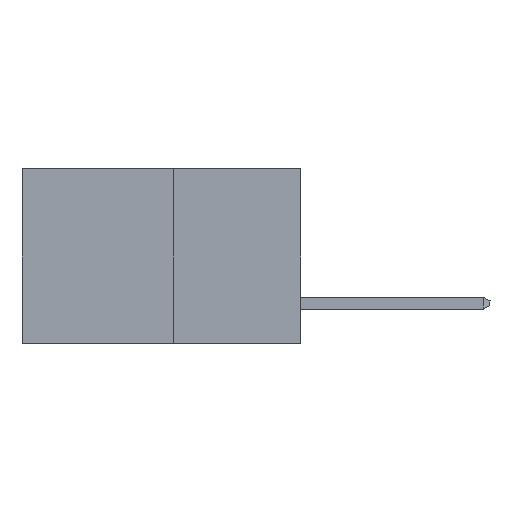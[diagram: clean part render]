
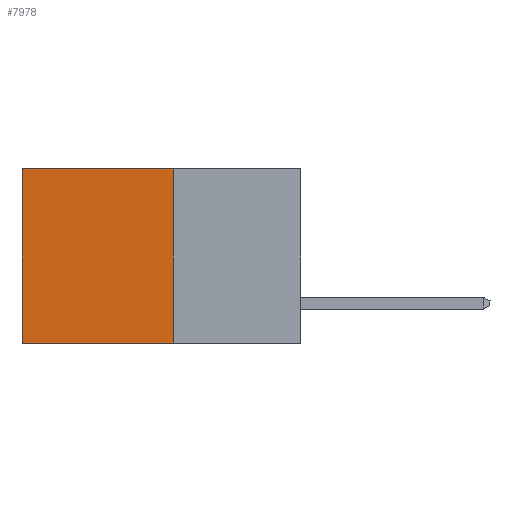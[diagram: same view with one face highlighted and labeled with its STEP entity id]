
A CAD part, left-side view. The second image highlights one B-rep face of the part: STEP entity #7978.
In plain terms, the highlighted planar face has unit normal (-1, 0, 0).
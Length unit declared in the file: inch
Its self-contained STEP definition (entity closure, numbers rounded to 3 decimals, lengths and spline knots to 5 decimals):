
#73 = DIRECTION ( 'NONE',  ( 0., 0., -1. ) ) ;
#95 = EDGE_CURVE ( 'NONE', #4328, #338, #3248, .T. ) ;
#338 = VERTEX_POINT ( 'NONE', #5758 ) ;
#767 = CARTESIAN_POINT ( 'NONE',  ( 0.277, 0.27, 0. ) ) ;
#974 = VERTEX_POINT ( 'NONE', #5939 ) ;
#1022 = LINE ( 'NONE', #767, #6260 ) ;
#1115 = LINE ( 'NONE', #7051, #4926 ) ;
#1718 = VERTEX_POINT ( 'NONE', #2496 ) ;
#2496 = CARTESIAN_POINT ( 'NONE',  ( 0.277, 0.59, 0. ) ) ;
#2800 = ORIENTED_EDGE ( 'NONE', *, *, #3115, .F. ) ;
#3115 = EDGE_CURVE ( 'NONE', #974, #4328, #1115, .T. ) ;
#3248 = LINE ( 'NONE', #6952, #6782 ) ;
#3275 = FACE_OUTER_BOUND ( 'NONE', #4754, .T. ) ;
#3795 = ORIENTED_EDGE ( 'NONE', *, *, #7130, .T. ) ;
#3857 = PLANE ( 'NONE',  #6784 ) ;
#4147 = CARTESIAN_POINT ( 'NONE',  ( 0.277, 0.59, -0.37 ) ) ;
#4328 = VERTEX_POINT ( 'NONE', #5882 ) ;
#4445 = ORIENTED_EDGE ( 'NONE', *, *, #8864, .T. ) ;
#4510 = VECTOR ( 'NONE', #6279, 39.37008 ) ;
#4560 = DIRECTION ( 'NONE',  ( 0., 0., -1. ) ) ;
#4754 = EDGE_LOOP ( 'NONE', ( #3795, #5561, #2800, #4445 ) ) ;
#4926 = VECTOR ( 'NONE', #73, 39.37008 ) ;
#5561 = ORIENTED_EDGE ( 'NONE', *, *, #95, .F. ) ;
#5758 = CARTESIAN_POINT ( 'NONE',  ( 0.277, 0.59, -0.37 ) ) ;
#5882 = CARTESIAN_POINT ( 'NONE',  ( 0.277, 0.27, -0.37 ) ) ;
#5939 = CARTESIAN_POINT ( 'NONE',  ( 0.277, 0.27, 0. ) ) ;
#5952 = CARTESIAN_POINT ( 'NONE',  ( 0.277, 0.27, -0.37 ) ) ;
#6260 = VECTOR ( 'NONE', #7828, 39.37008 ) ;
#6279 = DIRECTION ( 'NONE',  ( 0., 0., -1. ) ) ;
#6382 = LINE ( 'NONE', #4147, #4510 ) ;
#6782 = VECTOR ( 'NONE', #7094, 39.37008 ) ;
#6784 = AXIS2_PLACEMENT_3D ( 'NONE', #5952, #8725, #4560 ) ;
#6952 = CARTESIAN_POINT ( 'NONE',  ( 0.277, 0.27, -0.37 ) ) ;
#7051 = CARTESIAN_POINT ( 'NONE',  ( 0.277, 0.27, -0.37 ) ) ;
#7094 = DIRECTION ( 'NONE',  ( 0., 1., 0. ) ) ;
#7130 = EDGE_CURVE ( 'NONE', #1718, #338, #6382, .T. ) ;
#7828 = DIRECTION ( 'NONE',  ( 0., 1., 0. ) ) ;
#7978 = ADVANCED_FACE ( 'NONE', ( #3275 ), #3857, .F. ) ;
#8725 = DIRECTION ( 'NONE',  ( 1., 0., 0. ) ) ;
#8864 = EDGE_CURVE ( 'NONE', #974, #1718, #1022, .T. ) ;
